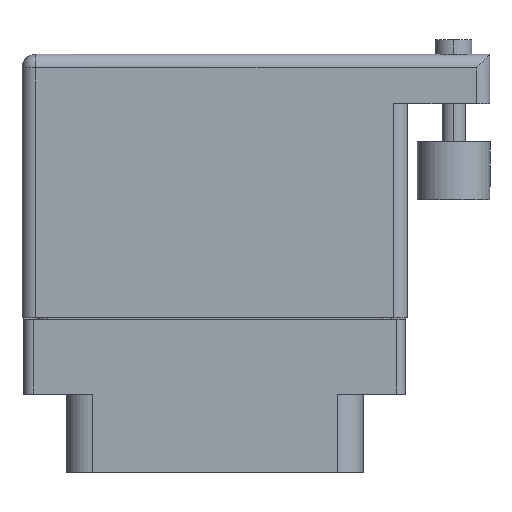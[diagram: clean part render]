
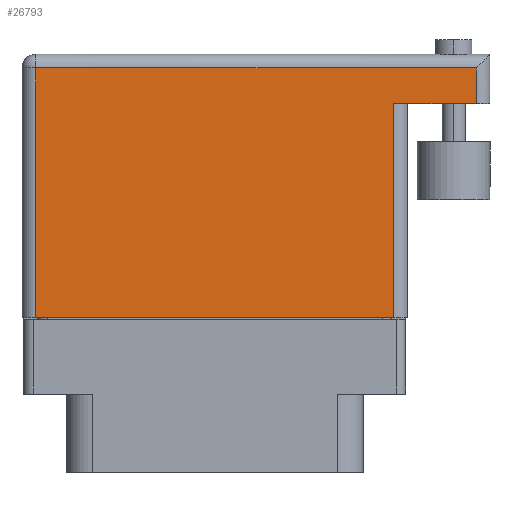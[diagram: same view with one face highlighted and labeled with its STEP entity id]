
A CAD part, front view. The second image highlights one B-rep face of the part: STEP entity #26793.
In plain terms, the highlighted face is planar.
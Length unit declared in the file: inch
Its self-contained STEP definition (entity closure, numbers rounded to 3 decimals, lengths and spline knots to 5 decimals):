
#702 = LINE ( 'NONE', #22082, #9290 ) ;
#1292 = DIRECTION ( 'NONE',  ( 0., 1., 0. ) ) ;
#3053 = DIRECTION ( 'NONE',  ( -1., 0., 0. ) ) ;
#3248 = CARTESIAN_POINT ( 'NONE',  ( -0.6625, 0.806, 0.3575 ) ) ;
#3255 = LINE ( 'NONE', #15228, #12543 ) ;
#3562 = DIRECTION ( 'NONE',  ( -1., 0., 0. ) ) ;
#4605 = ORIENTED_EDGE ( 'NONE', *, *, #24800, .T. ) ;
#5107 = DIRECTION ( 'NONE',  ( 0., 1., 0. ) ) ;
#7383 = VERTEX_POINT ( 'NONE', #28493 ) ;
#7797 = EDGE_CURVE ( 'NONE', #7383, #23337, #702, .T. ) ;
#8006 = VERTEX_POINT ( 'NONE', #30314 ) ;
#9080 = FACE_OUTER_BOUND ( 'NONE', #27249, .T. ) ;
#9290 = VECTOR ( 'NONE', #29267, 39.37008 ) ;
#10611 = VERTEX_POINT ( 'NONE', #29656 ) ;
#10797 = LINE ( 'NONE', #29937, #24621 ) ;
#11112 = CARTESIAN_POINT ( 'NONE',  ( -0.6155, -0.1, 0.3575 ) ) ;
#12413 = CARTESIAN_POINT ( 'NONE',  ( -0.6625, 0.759, 0.3575 ) ) ;
#12543 = VECTOR ( 'NONE', #1292, 39.37008 ) ;
#14551 = CARTESIAN_POINT ( 'NONE',  ( 0.6155, 0.636, 0.3575 ) ) ;
#14880 = EDGE_CURVE ( 'NONE', #23337, #8006, #25673, .T. ) ;
#15228 = CARTESIAN_POINT ( 'NONE',  ( 0.8995, 0.806, 0.3575 ) ) ;
#15501 = EDGE_CURVE ( 'NONE', #22915, #20172, #3255, .T. ) ;
#16533 = ORIENTED_EDGE ( 'NONE', *, *, #25731, .T. ) ;
#17075 = ORIENTED_EDGE ( 'NONE', *, *, #7797, .T. ) ;
#17644 = AXIS2_PLACEMENT_3D ( 'NONE', #3248, #17749, #3562 ) ;
#17749 = DIRECTION ( 'NONE',  ( 0., 0., -1. ) ) ;
#18695 = DIRECTION ( 'NONE',  ( 0., -1., 0. ) ) ;
#19742 = VECTOR ( 'NONE', #18695, 39.37008 ) ;
#20172 = VERTEX_POINT ( 'NONE', #25151 ) ;
#20621 = ORIENTED_EDGE ( 'NONE', *, *, #15501, .T. ) ;
#21248 = LINE ( 'NONE', #11112, #19742 ) ;
#22082 = CARTESIAN_POINT ( 'NONE',  ( -0.6625, -0.1, 0.3575 ) ) ;
#22102 = VECTOR ( 'NONE', #3053, 39.37008 ) ;
#22915 = VERTEX_POINT ( 'NONE', #25516 ) ;
#23337 = VERTEX_POINT ( 'NONE', #29848 ) ;
#23985 = LINE ( 'NONE', #12413, #22102 ) ;
#24621 = VECTOR ( 'NONE', #27439, 39.37008 ) ;
#24732 = ORIENTED_EDGE ( 'NONE', *, *, #14880, .T. ) ;
#24800 = EDGE_CURVE ( 'NONE', #10611, #7383, #21248, .T. ) ;
#25151 = CARTESIAN_POINT ( 'NONE',  ( 0.8995, 0.759, 0.3575 ) ) ;
#25516 = CARTESIAN_POINT ( 'NONE',  ( 0.8995, 0.636, 0.3575 ) ) ;
#25673 = LINE ( 'NONE', #14551, #27150 ) ;
#25731 = EDGE_CURVE ( 'NONE', #20172, #10611, #23985, .T. ) ;
#26793 = ADVANCED_FACE ( 'NONE', ( #9080 ), #29781, .F. ) ;
#27150 = VECTOR ( 'NONE', #5107, 39.37008 ) ;
#27249 = EDGE_LOOP ( 'NONE', ( #17075, #24732, #28466, #20621, #16533, #4605 ) ) ;
#27439 = DIRECTION ( 'NONE',  ( -1., 0., 0. ) ) ;
#28429 = EDGE_CURVE ( 'NONE', #22915, #8006, #10797, .T. ) ;
#28466 = ORIENTED_EDGE ( 'NONE', *, *, #28429, .F. ) ;
#28493 = CARTESIAN_POINT ( 'NONE',  ( -0.6155, -0.1, 0.3575 ) ) ;
#29267 = DIRECTION ( 'NONE',  ( 1., 0., 0. ) ) ;
#29656 = CARTESIAN_POINT ( 'NONE',  ( -0.6155, 0.759, 0.3575 ) ) ;
#29781 = PLANE ( 'NONE',  #17644 ) ;
#29848 = CARTESIAN_POINT ( 'NONE',  ( 0.6155, -0.1, 0.3575 ) ) ;
#29937 = CARTESIAN_POINT ( 'NONE',  ( 0.9465, 0.636, 0.3575 ) ) ;
#30314 = CARTESIAN_POINT ( 'NONE',  ( 0.6155, 0.636, 0.3575 ) ) ;
